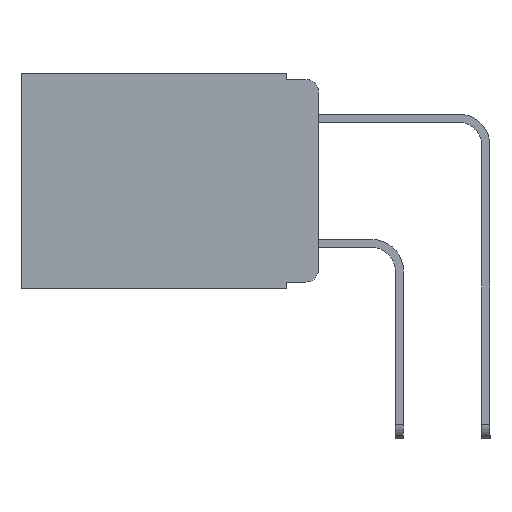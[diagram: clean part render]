
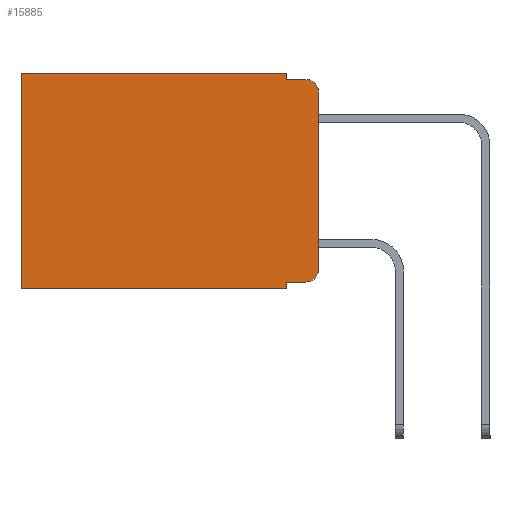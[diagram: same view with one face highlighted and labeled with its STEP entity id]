
A CAD part, left-side view. The second image highlights one B-rep face of the part: STEP entity #15885.
In plain terms, the highlighted planar face has unit normal (-1, 0, 0).
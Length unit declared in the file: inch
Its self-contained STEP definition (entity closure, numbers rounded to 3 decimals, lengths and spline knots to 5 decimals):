
#1732 = DIRECTION ( 'NONE',  ( 0., 1., 0. ) ) ;
#1863 = VERTEX_POINT ( 'NONE', #17610 ) ;
#2221 = VECTOR ( 'NONE', #2337, 39.37008 ) ;
#2239 = VERTEX_POINT ( 'NONE', #17271 ) ;
#2337 = DIRECTION ( 'NONE',  ( 0., 0., -1. ) ) ;
#2473 = VERTEX_POINT ( 'NONE', #16044 ) ;
#2714 = CARTESIAN_POINT ( 'NONE',  ( 0.298, 0., -0.313 ) ) ;
#2866 = DIRECTION ( 'NONE',  ( -1., 0., 0. ) ) ;
#3287 = EDGE_LOOP ( 'NONE', ( #15841, #14961, #14657, #14165, #13239, #15611, #21826, #10387, #15049, #8257 ) ) ;
#3329 = VECTOR ( 'NONE', #12456, 39.37008 ) ;
#4041 = EDGE_CURVE ( 'NONE', #22796, #2473, #18982, .T. ) ;
#4108 = AXIS2_PLACEMENT_3D ( 'NONE', #20301, #9200, #22120 ) ;
#4221 = VECTOR ( 'NONE', #22396, 39.37008 ) ;
#4305 = CARTESIAN_POINT ( 'NONE',  ( 0.298, 0.051, -0.333 ) ) ;
#4657 = EDGE_CURVE ( 'NONE', #14298, #2239, #6680, .T. ) ;
#5185 = EDGE_CURVE ( 'NONE', #13886, #12555, #9301, .T. ) ;
#5533 = CIRCLE ( 'NONE', #10401, 0.02 ) ;
#6077 = VECTOR ( 'NONE', #18542, 39.37008 ) ;
#6318 = CARTESIAN_POINT ( 'NONE',  ( 0.298, 0., 0. ) ) ;
#6680 = LINE ( 'NONE', #23881, #6077 ) ;
#7050 = CARTESIAN_POINT ( 'NONE',  ( 0.298, 0.051, 0. ) ) ;
#7176 = AXIS2_PLACEMENT_3D ( 'NONE', #6318, #22976, #12009 ) ;
#7527 = CARTESIAN_POINT ( 'NONE',  ( 0.298, 0., -0.343 ) ) ;
#7791 = CARTESIAN_POINT ( 'NONE',  ( 0.298, 0.051, -0.343 ) ) ;
#7805 = LINE ( 'NONE', #4305, #22018 ) ;
#7957 = CARTESIAN_POINT ( 'NONE',  ( 0.298, 0.02, -0.01 ) ) ;
#7996 = VECTOR ( 'NONE', #10959, 39.37008 ) ;
#8004 = CARTESIAN_POINT ( 'NONE',  ( 0.298, 0.051, 0. ) ) ;
#8257 = ORIENTED_EDGE ( 'NONE', *, *, #16219, .T. ) ;
#9015 = EDGE_CURVE ( 'NONE', #1863, #12555, #5533, .T. ) ;
#9200 = DIRECTION ( 'NONE',  ( -1., 0., 0. ) ) ;
#9301 = LINE ( 'NONE', #18701, #4221 ) ;
#9370 = EDGE_CURVE ( 'NONE', #1863, #19238, #21544, .T. ) ;
#10130 = PLANE ( 'NONE',  #7176 ) ;
#10387 = ORIENTED_EDGE ( 'NONE', *, *, #13253, .F. ) ;
#10401 = AXIS2_PLACEMENT_3D ( 'NONE', #14230, #2866, #16124 ) ;
#10581 = CARTESIAN_POINT ( 'NONE',  ( 0.298, 0.051, 0. ) ) ;
#10959 = DIRECTION ( 'NONE',  ( 0., 0., -1. ) ) ;
#11540 = CARTESIAN_POINT ( 'NONE',  ( 0.298, 0., 0. ) ) ;
#11701 = CARTESIAN_POINT ( 'NONE',  ( 0.298, 0.051, -0.01 ) ) ;
#11749 = VECTOR ( 'NONE', #22538, 39.37008 ) ;
#11821 = VERTEX_POINT ( 'NONE', #17073 ) ;
#11879 = CIRCLE ( 'NONE', #4108, 0.02 ) ;
#12009 = DIRECTION ( 'NONE',  ( 0., 0., -1. ) ) ;
#12456 = DIRECTION ( 'NONE',  ( 0., 0., -1. ) ) ;
#12555 = VERTEX_POINT ( 'NONE', #7957 ) ;
#13239 = ORIENTED_EDGE ( 'NONE', *, *, #4657, .T. ) ;
#13253 = EDGE_CURVE ( 'NONE', #11821, #22796, #17363, .T. ) ;
#13429 = FACE_OUTER_BOUND ( 'NONE', #3287, .T. ) ;
#13886 = VERTEX_POINT ( 'NONE', #11701 ) ;
#14050 = VECTOR ( 'NONE', #1732, 39.37008 ) ;
#14165 = ORIENTED_EDGE ( 'NONE', *, *, #20653, .F. ) ;
#14230 = CARTESIAN_POINT ( 'NONE',  ( 0.298, 0.02, -0.03 ) ) ;
#14298 = VERTEX_POINT ( 'NONE', #7050 ) ;
#14657 = ORIENTED_EDGE ( 'NONE', *, *, #5185, .F. ) ;
#14691 = CARTESIAN_POINT ( 'NONE',  ( 0.298, 0.473, 0. ) ) ;
#14961 = ORIENTED_EDGE ( 'NONE', *, *, #9015, .T. ) ;
#15049 = ORIENTED_EDGE ( 'NONE', *, *, #21121, .T. ) ;
#15611 = ORIENTED_EDGE ( 'NONE', *, *, #16994, .T. ) ;
#15656 = CARTESIAN_POINT ( 'NONE',  ( 0.298, 0.02, -0.333 ) ) ;
#15841 = ORIENTED_EDGE ( 'NONE', *, *, #9370, .F. ) ;
#15885 = ADVANCED_FACE ( 'NONE', ( #13429 ), #10130, .F. ) ;
#16044 = CARTESIAN_POINT ( 'NONE',  ( 0.298, 0.473, -0.343 ) ) ;
#16124 = DIRECTION ( 'NONE',  ( 0., 0., -1. ) ) ;
#16219 = EDGE_CURVE ( 'NONE', #22254, #19238, #11879, .T. ) ;
#16994 = EDGE_CURVE ( 'NONE', #2239, #2473, #23303, .T. ) ;
#17073 = CARTESIAN_POINT ( 'NONE',  ( 0.298, 0.051, -0.333 ) ) ;
#17271 = CARTESIAN_POINT ( 'NONE',  ( 0.298, 0.473, 0. ) ) ;
#17363 = LINE ( 'NONE', #8004, #2221 ) ;
#17610 = CARTESIAN_POINT ( 'NONE',  ( 0.298, 0., -0.03 ) ) ;
#18542 = DIRECTION ( 'NONE',  ( 0., 1., 0. ) ) ;
#18701 = CARTESIAN_POINT ( 'NONE',  ( 0.298, 0.051, -0.01 ) ) ;
#18941 = LINE ( 'NONE', #10581, #3329 ) ;
#18982 = LINE ( 'NONE', #7527, #14050 ) ;
#19238 = VERTEX_POINT ( 'NONE', #2714 ) ;
#20301 = CARTESIAN_POINT ( 'NONE',  ( 0.298, 0.02, -0.313 ) ) ;
#20653 = EDGE_CURVE ( 'NONE', #14298, #13886, #18941, .T. ) ;
#21121 = EDGE_CURVE ( 'NONE', #11821, #22254, #7805, .T. ) ;
#21544 = LINE ( 'NONE', #11540, #11749 ) ;
#21826 = ORIENTED_EDGE ( 'NONE', *, *, #4041, .F. ) ;
#22018 = VECTOR ( 'NONE', #22840, 39.37008 ) ;
#22120 = DIRECTION ( 'NONE',  ( 0., 0., -1. ) ) ;
#22254 = VERTEX_POINT ( 'NONE', #15656 ) ;
#22396 = DIRECTION ( 'NONE',  ( 0., -1., 0. ) ) ;
#22538 = DIRECTION ( 'NONE',  ( 0., 0., -1. ) ) ;
#22796 = VERTEX_POINT ( 'NONE', #7791 ) ;
#22840 = DIRECTION ( 'NONE',  ( 0., -1., 0. ) ) ;
#22976 = DIRECTION ( 'NONE',  ( 1., 0., 0. ) ) ;
#23303 = LINE ( 'NONE', #14691, #7996 ) ;
#23881 = CARTESIAN_POINT ( 'NONE',  ( 0.298, 0., 0. ) ) ;
